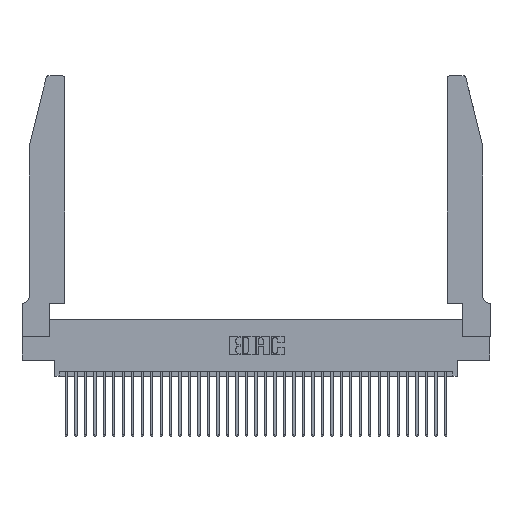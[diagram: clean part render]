
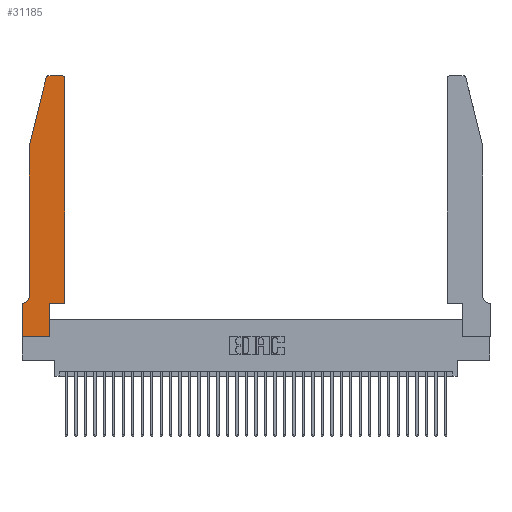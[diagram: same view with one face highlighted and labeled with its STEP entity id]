
A CAD part, top view. The second image highlights one B-rep face of the part: STEP entity #31185.
In plain terms, the highlighted planar face has unit normal (0, 0, 1).
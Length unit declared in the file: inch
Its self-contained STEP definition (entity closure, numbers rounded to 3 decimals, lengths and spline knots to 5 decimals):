
#311 = EDGE_CURVE ( 'NONE', #18505, #12822, #35311, .T. ) ;
#487 = VECTOR ( 'NONE', #13182, 39.37008 ) ;
#613 = VECTOR ( 'NONE', #27441, 39.37008 ) ;
#1333 = DIRECTION ( 'NONE',  ( 1., 0., 0. ) ) ;
#1380 = EDGE_CURVE ( 'NONE', #12822, #19554, #1534, .T. ) ;
#1534 = LINE ( 'NONE', #30317, #613 ) ;
#1618 = VECTOR ( 'NONE', #18646, 39.37008 ) ;
#2477 = LINE ( 'NONE', #13031, #17026 ) ;
#2504 = ORIENTED_EDGE ( 'NONE', *, *, #29087, .T. ) ;
#2530 = CARTESIAN_POINT ( 'NONE',  ( 0.0755, 2., 0.37 ) ) ;
#2988 = DIRECTION ( 'NONE',  ( 0., 0., 1. ) ) ;
#2996 = AXIS2_PLACEMENT_3D ( 'NONE', #20368, #2988, #23262 ) ;
#3237 = VERTEX_POINT ( 'NONE', #9394 ) ;
#3784 = CARTESIAN_POINT ( 'NONE',  ( 0.4505, 2.72, 0.37 ) ) ;
#4158 = CARTESIAN_POINT ( 'NONE',  ( 0.2605, 2.75, 0.37 ) ) ;
#4537 = CARTESIAN_POINT ( 'NONE',  ( 0.0055, 0.42, 0.37 ) ) ;
#5215 = VECTOR ( 'NONE', #12069, 39.37008 ) ;
#5612 = CARTESIAN_POINT ( 'NONE',  ( 0.0755, 0.42, 0.37 ) ) ;
#6056 = CARTESIAN_POINT ( 'NONE',  ( 0.4505, 0.35, 0.37 ) ) ;
#6350 = PLANE ( 'NONE',  #24119 ) ;
#6514 = ORIENTED_EDGE ( 'NONE', *, *, #36251, .T. ) ;
#6744 = VERTEX_POINT ( 'NONE', #31180 ) ;
#6767 = ORIENTED_EDGE ( 'NONE', *, *, #311, .T. ) ;
#7073 = VECTOR ( 'NONE', #27451, 39.37008 ) ;
#7594 = EDGE_CURVE ( 'NONE', #23047, #24503, #25709, .T. ) ;
#8205 = CARTESIAN_POINT ( 'NONE',  ( 0.25487, 2.72718, 0.37 ) ) ;
#8282 = LINE ( 'NONE', #17245, #23659 ) ;
#9078 = EDGE_CURVE ( 'NONE', #24503, #15823, #31385, .T. ) ;
#9394 = CARTESIAN_POINT ( 'NONE',  ( 0., 0., 0.37 ) ) ;
#9505 = VECTOR ( 'NONE', #20006, 39.37008 ) ;
#9891 = CARTESIAN_POINT ( 'NONE',  ( 0.0055, 0.35, 0.37 ) ) ;
#12069 = DIRECTION ( 'NONE',  ( 0., 1., 0. ) ) ;
#12365 = AXIS2_PLACEMENT_3D ( 'NONE', #4537, #18274, #18168 ) ;
#12474 = DIRECTION ( 'NONE',  ( 0., 0., 1. ) ) ;
#12822 = VERTEX_POINT ( 'NONE', #9891 ) ;
#13031 = CARTESIAN_POINT ( 'NONE',  ( 0.0755, 2., 0.37 ) ) ;
#13093 = VECTOR ( 'NONE', #22093, 39.37008 ) ;
#13182 = DIRECTION ( 'NONE',  ( 0., -1., 0. ) ) ;
#14098 = LINE ( 'NONE', #30410, #487 ) ;
#14131 = EDGE_CURVE ( 'NONE', #3237, #6744, #30110, .T. ) ;
#14881 = CARTESIAN_POINT ( 'NONE',  ( 0.284, 2.75, 0.37 ) ) ;
#15222 = EDGE_CURVE ( 'NONE', #27470, #18505, #2477, .T. ) ;
#15823 = VERTEX_POINT ( 'NONE', #14881 ) ;
#15891 = CARTESIAN_POINT ( 'NONE',  ( 0., 0.35, 0.37 ) ) ;
#16751 = CIRCLE ( 'NONE', #35157, 0.03 ) ;
#17026 = VECTOR ( 'NONE', #26889, 39.37008 ) ;
#17130 = VERTEX_POINT ( 'NONE', #35325 ) ;
#17245 = CARTESIAN_POINT ( 'NONE',  ( 0.2865, 0.35, 0.37 ) ) ;
#17256 = LINE ( 'NONE', #2530, #9505 ) ;
#18168 = DIRECTION ( 'NONE',  ( -1., 0., 0. ) ) ;
#18274 = DIRECTION ( 'NONE',  ( 0., 0., -1. ) ) ;
#18505 = VERTEX_POINT ( 'NONE', #5612 ) ;
#18646 = DIRECTION ( 'NONE',  ( -1., 0., 0. ) ) ;
#18706 = DIRECTION ( 'NONE',  ( 0., 0., 1. ) ) ;
#19196 = CARTESIAN_POINT ( 'NONE',  ( 0.4505, 0.35, 0.37 ) ) ;
#19554 = VERTEX_POINT ( 'NONE', #15891 ) ;
#20006 = DIRECTION ( 'NONE',  ( -0.239, -0.971, 0. ) ) ;
#20368 = CARTESIAN_POINT ( 'NONE',  ( 0.4205, 2.72, 0.37 ) ) ;
#20845 = ORIENTED_EDGE ( 'NONE', *, *, #1380, .T. ) ;
#21562 = LINE ( 'NONE', #26443, #5215 ) ;
#21746 = ORIENTED_EDGE ( 'NONE', *, *, #7594, .T. ) ;
#22093 = DIRECTION ( 'NONE',  ( 1., 0., 0. ) ) ;
#22934 = EDGE_CURVE ( 'NONE', #28520, #23047, #21562, .T. ) ;
#23047 = VERTEX_POINT ( 'NONE', #3784 ) ;
#23262 = DIRECTION ( 'NONE',  ( 1., 0., 0. ) ) ;
#23659 = VECTOR ( 'NONE', #34334, 39.37008 ) ;
#24119 = AXIS2_PLACEMENT_3D ( 'NONE', #29707, #12474, #32565 ) ;
#24503 = VERTEX_POINT ( 'NONE', #33193 ) ;
#24584 = CARTESIAN_POINT ( 'NONE',  ( 0., 0., 0.37 ) ) ;
#24623 = CARTESIAN_POINT ( 'NONE',  ( 0.0755, 2., 0.37 ) ) ;
#25709 = CIRCLE ( 'NONE', #2996, 0.03 ) ;
#26443 = CARTESIAN_POINT ( 'NONE',  ( 0.4505, 0.35, 0.37 ) ) ;
#26889 = DIRECTION ( 'NONE',  ( 0., -1., 0. ) ) ;
#27057 = VERTEX_POINT ( 'NONE', #8205 ) ;
#27441 = DIRECTION ( 'NONE',  ( -1., 0., 0. ) ) ;
#27451 = DIRECTION ( 'NONE',  ( 1., 0., 0. ) ) ;
#27470 = VERTEX_POINT ( 'NONE', #24623 ) ;
#27540 = ORIENTED_EDGE ( 'NONE', *, *, #22934, .T. ) ;
#27748 = ORIENTED_EDGE ( 'NONE', *, *, #9078, .T. ) ;
#28451 = ORIENTED_EDGE ( 'NONE', *, *, #15222, .T. ) ;
#28520 = VERTEX_POINT ( 'NONE', #6056 ) ;
#29087 = EDGE_CURVE ( 'NONE', #6744, #17130, #8282, .T. ) ;
#29292 = LINE ( 'NONE', #19196, #13093 ) ;
#29707 = CARTESIAN_POINT ( 'NONE',  ( 0., 0.35, 0.37 ) ) ;
#30051 = EDGE_CURVE ( 'NONE', #19554, #3237, #14098, .T. ) ;
#30110 = LINE ( 'NONE', #24584, #7073 ) ;
#30317 = CARTESIAN_POINT ( 'NONE',  ( 0.0755, 0.35, 0.37 ) ) ;
#30410 = CARTESIAN_POINT ( 'NONE',  ( 0., 0., 0.37 ) ) ;
#31180 = CARTESIAN_POINT ( 'NONE',  ( 0.2865, 0., 0.37 ) ) ;
#31185 = ADVANCED_FACE ( 'NONE', ( #37152 ), #6350, .T. ) ;
#31334 = ORIENTED_EDGE ( 'NONE', *, *, #30051, .T. ) ;
#31385 = LINE ( 'NONE', #4158, #1618 ) ;
#31791 = ORIENTED_EDGE ( 'NONE', *, *, #14131, .T. ) ;
#32380 = ORIENTED_EDGE ( 'NONE', *, *, #36400, .T. ) ;
#32565 = DIRECTION ( 'NONE',  ( 1., 0., 0. ) ) ;
#33193 = CARTESIAN_POINT ( 'NONE',  ( 0.4205, 2.75, 0.37 ) ) ;
#34334 = DIRECTION ( 'NONE',  ( 0., 1., 0. ) ) ;
#35022 = EDGE_LOOP ( 'NONE', ( #27748, #6514, #37111, #28451, #6767, #20845, #31334, #31791, #2504, #32380, #27540, #21746 ) ) ;
#35157 = AXIS2_PLACEMENT_3D ( 'NONE', #35783, #18706, #1333 ) ;
#35311 = CIRCLE ( 'NONE', #12365, 0.07 ) ;
#35325 = CARTESIAN_POINT ( 'NONE',  ( 0.2865, 0.35, 0.37 ) ) ;
#35574 = EDGE_CURVE ( 'NONE', #27057, #27470, #17256, .T. ) ;
#35783 = CARTESIAN_POINT ( 'NONE',  ( 0.284, 2.72, 0.37 ) ) ;
#36251 = EDGE_CURVE ( 'NONE', #15823, #27057, #16751, .T. ) ;
#36400 = EDGE_CURVE ( 'NONE', #17130, #28520, #29292, .T. ) ;
#37111 = ORIENTED_EDGE ( 'NONE', *, *, #35574, .T. ) ;
#37152 = FACE_OUTER_BOUND ( 'NONE', #35022, .T. ) ;
